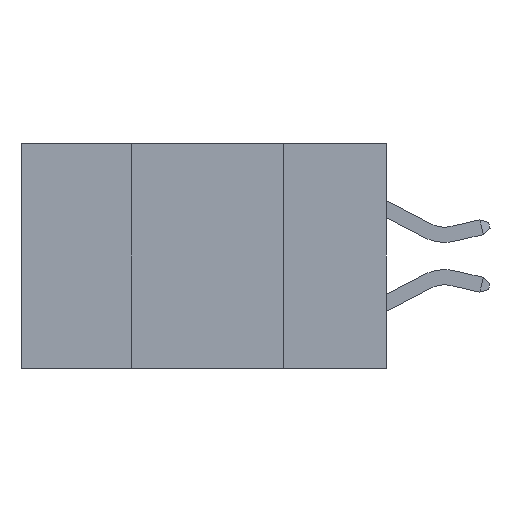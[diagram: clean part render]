
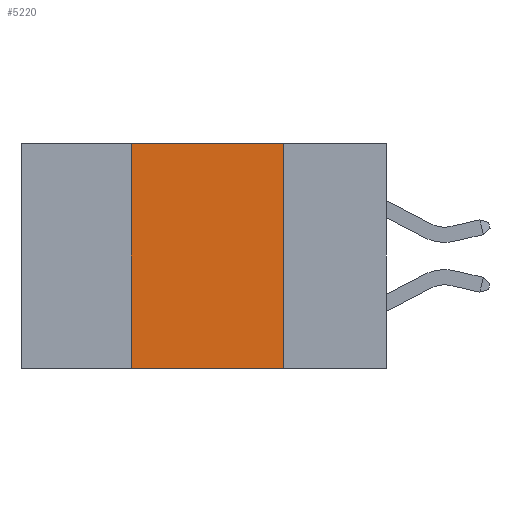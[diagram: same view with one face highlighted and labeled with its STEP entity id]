
A CAD part, left-side view. The second image highlights one B-rep face of the part: STEP entity #5220.
In plain terms, the highlighted planar face has unit normal (-1, 0, 0).
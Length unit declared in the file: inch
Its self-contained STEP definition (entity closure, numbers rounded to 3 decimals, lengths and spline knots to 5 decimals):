
#329 = LINE ( 'NONE', #9791, #1114 ) ;
#849 = CARTESIAN_POINT ( 'NONE',  ( 0., 0.6, 0. ) ) ;
#1114 = VECTOR ( 'NONE', #11209, 39.37008 ) ;
#1988 = DIRECTION ( 'NONE',  ( 0., 0., -1. ) ) ;
#2140 = CARTESIAN_POINT ( 'NONE',  ( 0., 0.6, 0. ) ) ;
#2209 = DIRECTION ( 'NONE',  ( 0., 0., 1. ) ) ;
#2456 = VERTEX_POINT ( 'NONE', #12888 ) ;
#2472 = EDGE_CURVE ( 'NONE', #4072, #3068, #11703, .T. ) ;
#2478 = CARTESIAN_POINT ( 'NONE',  ( 0., 0.6, -0.37 ) ) ;
#3068 = VERTEX_POINT ( 'NONE', #8272 ) ;
#3331 = VECTOR ( 'NONE', #2209, 39.37008 ) ;
#3994 = ORIENTED_EDGE ( 'NONE', *, *, #6768, .F. ) ;
#4072 = VERTEX_POINT ( 'NONE', #7831 ) ;
#4150 = ORIENTED_EDGE ( 'NONE', *, *, #2472, .F. ) ;
#4306 = LINE ( 'NONE', #849, #5895 ) ;
#5220 = ADVANCED_FACE ( 'NONE', ( #12893 ), #11634, .F. ) ;
#5895 = VECTOR ( 'NONE', #9061, 39.37008 ) ;
#6664 = CARTESIAN_POINT ( 'NONE',  ( 0., 0.17, -0.37 ) ) ;
#6768 = EDGE_CURVE ( 'NONE', #2456, #11715, #329, .T. ) ;
#6937 = EDGE_CURVE ( 'NONE', #3068, #2456, #4306, .T. ) ;
#7658 = ORIENTED_EDGE ( 'NONE', *, *, #13830, .T. ) ;
#7831 = CARTESIAN_POINT ( 'NONE',  ( 0., 0.42, -0.37 ) ) ;
#7983 = DIRECTION ( 'NONE',  ( 1., 0., 0. ) ) ;
#8214 = CARTESIAN_POINT ( 'NONE',  ( 0., 0.42, -0.37 ) ) ;
#8272 = CARTESIAN_POINT ( 'NONE',  ( 0., 0.42, 0. ) ) ;
#9061 = DIRECTION ( 'NONE',  ( 0., -1., 0. ) ) ;
#9483 = EDGE_LOOP ( 'NONE', ( #3994, #11636, #4150, #7658 ) ) ;
#9791 = CARTESIAN_POINT ( 'NONE',  ( 0., 0.17, -0.37 ) ) ;
#10868 = LINE ( 'NONE', #2478, #14450 ) ;
#11209 = DIRECTION ( 'NONE',  ( 0., 0., -1. ) ) ;
#11634 = PLANE ( 'NONE',  #12376 ) ;
#11636 = ORIENTED_EDGE ( 'NONE', *, *, #6937, .F. ) ;
#11703 = LINE ( 'NONE', #8214, #3331 ) ;
#11715 = VERTEX_POINT ( 'NONE', #6664 ) ;
#12287 = DIRECTION ( 'NONE',  ( 0., -1., 0. ) ) ;
#12376 = AXIS2_PLACEMENT_3D ( 'NONE', #2140, #7983, #1988 ) ;
#12888 = CARTESIAN_POINT ( 'NONE',  ( 0., 0.17, 0. ) ) ;
#12893 = FACE_OUTER_BOUND ( 'NONE', #9483, .T. ) ;
#13830 = EDGE_CURVE ( 'NONE', #4072, #11715, #10868, .T. ) ;
#14450 = VECTOR ( 'NONE', #12287, 39.37008 ) ;
